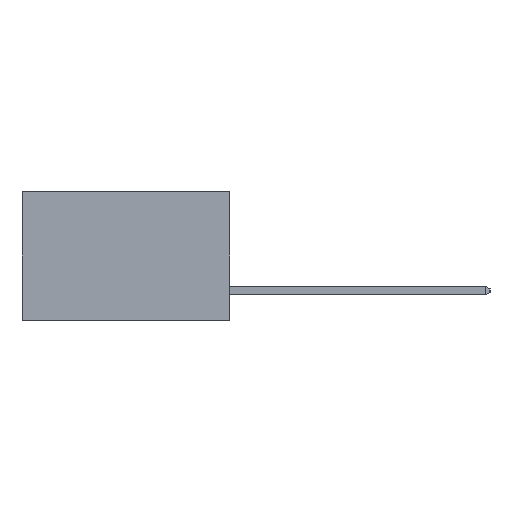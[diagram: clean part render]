
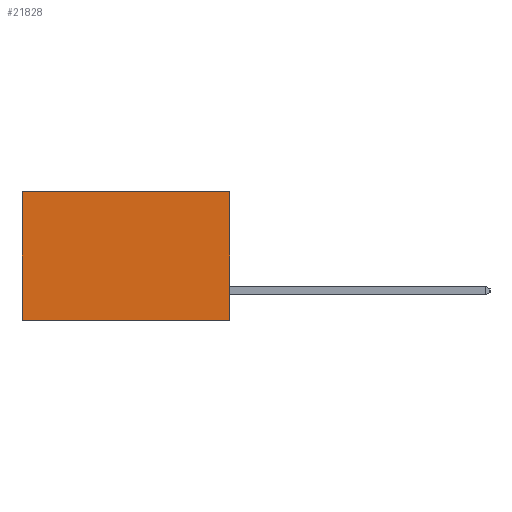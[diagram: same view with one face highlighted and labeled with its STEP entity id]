
A CAD part, left-side view. The second image highlights one B-rep face of the part: STEP entity #21828.
In plain terms, the highlighted planar face has unit normal (-1, 0, 0).
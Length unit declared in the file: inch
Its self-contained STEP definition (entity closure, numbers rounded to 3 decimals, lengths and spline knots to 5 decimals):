
#583 = CARTESIAN_POINT ( 'NONE',  ( 0.298, 0.6, -0.37 ) ) ;
#1449 = CARTESIAN_POINT ( 'NONE',  ( 0.298, 0., 0. ) ) ;
#2326 = ORIENTED_EDGE ( 'NONE', *, *, #20735, .F. ) ;
#2853 = LINE ( 'NONE', #14307, #8660 ) ;
#3195 = LINE ( 'NONE', #1449, #8981 ) ;
#4343 = EDGE_CURVE ( 'NONE', #23000, #29335, #16395, .T. ) ;
#8660 = VECTOR ( 'NONE', #21740, 39.37008 ) ;
#8981 = VECTOR ( 'NONE', #30667, 39.37008 ) ;
#9546 = EDGE_CURVE ( 'NONE', #21833, #23000, #3195, .T. ) ;
#10199 = AXIS2_PLACEMENT_3D ( 'NONE', #22708, #27475, #12912 ) ;
#10463 = PLANE ( 'NONE',  #10199 ) ;
#11964 = FACE_OUTER_BOUND ( 'NONE', #30695, .T. ) ;
#12420 = CARTESIAN_POINT ( 'NONE',  ( 0.298, 0., -0.37 ) ) ;
#12912 = DIRECTION ( 'NONE',  ( 0., 0., -1. ) ) ;
#13391 = VERTEX_POINT ( 'NONE', #15952 ) ;
#14307 = CARTESIAN_POINT ( 'NONE',  ( 0.298, 0., 0. ) ) ;
#14624 = ORIENTED_EDGE ( 'NONE', *, *, #4343, .T. ) ;
#15183 = CARTESIAN_POINT ( 'NONE',  ( 0.298, 0.6, 0. ) ) ;
#15629 = VECTOR ( 'NONE', #20584, 39.37008 ) ;
#15952 = CARTESIAN_POINT ( 'NONE',  ( 0.298, 0., -0.37 ) ) ;
#16395 = LINE ( 'NONE', #29046, #15629 ) ;
#19399 = EDGE_CURVE ( 'NONE', #21833, #13391, #2853, .T. ) ;
#20584 = DIRECTION ( 'NONE',  ( 0., 0., -1. ) ) ;
#20735 = EDGE_CURVE ( 'NONE', #13391, #29335, #26507, .T. ) ;
#20923 = ORIENTED_EDGE ( 'NONE', *, *, #9546, .T. ) ;
#21740 = DIRECTION ( 'NONE',  ( 0., 0., -1. ) ) ;
#21828 = ADVANCED_FACE ( 'NONE', ( #11964 ), #10463, .F. ) ;
#21833 = VERTEX_POINT ( 'NONE', #25110 ) ;
#22320 = DIRECTION ( 'NONE',  ( 0., 1., 0. ) ) ;
#22708 = CARTESIAN_POINT ( 'NONE',  ( 0.298, 0., 0. ) ) ;
#23000 = VERTEX_POINT ( 'NONE', #15183 ) ;
#25110 = CARTESIAN_POINT ( 'NONE',  ( 0.298, 0., 0. ) ) ;
#25756 = VECTOR ( 'NONE', #22320, 39.37008 ) ;
#26507 = LINE ( 'NONE', #12420, #25756 ) ;
#27475 = DIRECTION ( 'NONE',  ( 1., 0., 0. ) ) ;
#28001 = ORIENTED_EDGE ( 'NONE', *, *, #19399, .F. ) ;
#29046 = CARTESIAN_POINT ( 'NONE',  ( 0.298, 0.6, 0. ) ) ;
#29335 = VERTEX_POINT ( 'NONE', #583 ) ;
#30667 = DIRECTION ( 'NONE',  ( 0., 1., 0. ) ) ;
#30695 = EDGE_LOOP ( 'NONE', ( #14624, #2326, #28001, #20923 ) ) ;
